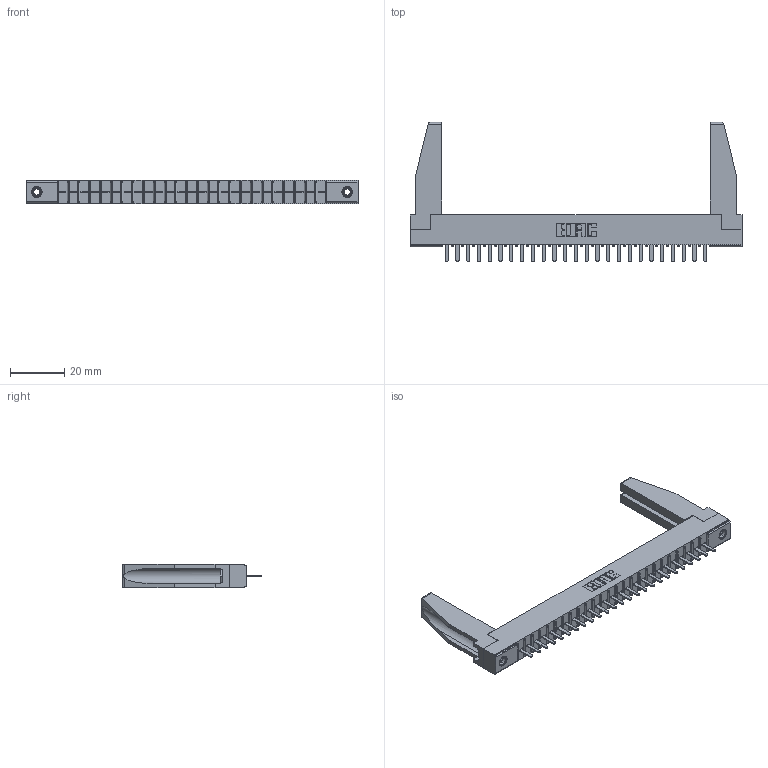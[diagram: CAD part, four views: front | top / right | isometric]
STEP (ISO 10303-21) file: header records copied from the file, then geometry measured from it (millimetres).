
FILE_DESCRIPTION (( 'STEP AP203' ), '1' );
FILE_NAME ('306-025-420-178.STEP', '2020-09-21T22:48:34', ( '' ), ( '' ), 'SwSTEP 2.0', 'SolidWorks 2020', '' );
FILE_SCHEMA (( 'CONFIG_CONTROL_DESIGN' ));
Length unit declared in the file: inch
Products named in the file (5): 307-220-078; 306 Part_.156 Dia; 306-025-420-178; 345-250-001_345-250-001-102; 306-290-001_120
Assembly tree (30 placements, depth 2):
  306-025-420-178
    306 Part_.156 Dia
    306-290-001_120  x25
    345-250-001_345-250-001-102  x2
    307-220-078  x2
Bounding box: 122.07 x 51.16 x 8.71 mm (x, y, z)
Volume: 12355 mm3; surface area: 16298.4 mm2
Topology: 30 solids, 30 shells, 1996 faces, 5571 edges, 3570 vertices
Faces by surface type: plane 1327, cylinder 553, sphere 100, cone 12, torus 4
Entity records: 27911 total; most frequent: CARTESIAN_POINT 4684, ORIENTED_EDGE 4600, DIRECTION 4572, EDGE_CURVE 2300, VECTOR 1792, LINE 1792, VERTEX_POINT 1460, AXIS2_PLACEMENT_3D 1390
